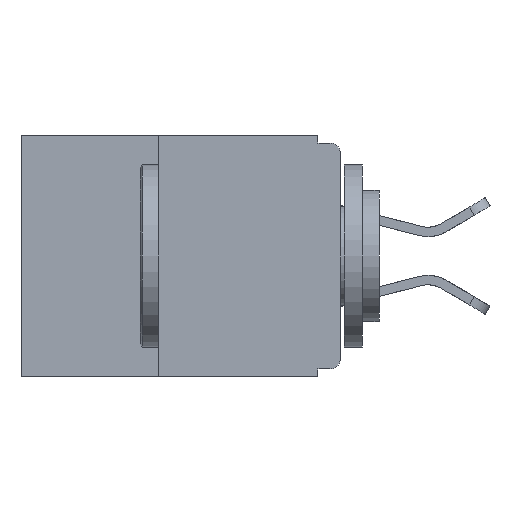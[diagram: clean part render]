
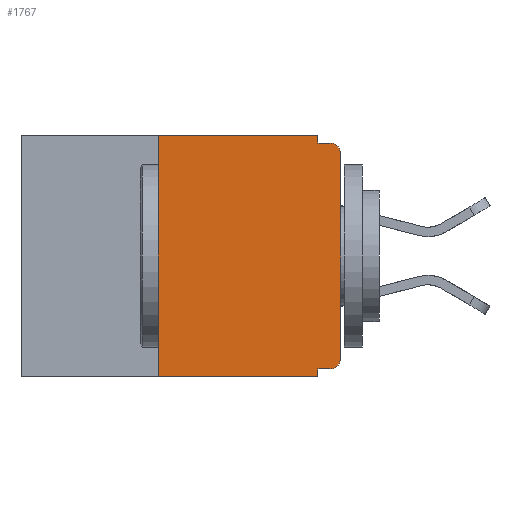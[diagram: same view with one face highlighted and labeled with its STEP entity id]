
A CAD part, left-side view. The second image highlights one B-rep face of the part: STEP entity #1767.
In plain terms, the highlighted planar face has unit normal (-1, 0, 0).
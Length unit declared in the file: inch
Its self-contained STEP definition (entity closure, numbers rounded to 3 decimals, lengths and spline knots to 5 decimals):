
#388 = ORIENTED_EDGE ( 'NONE', *, *, #21669, .T. ) ;
#803 = AXIS2_PLACEMENT_3D ( 'NONE', #18726, #20432, #6730 ) ;
#1104 = EDGE_CURVE ( 'NONE', #9653, #21299, #22819, .T. ) ;
#1432 = CARTESIAN_POINT ( 'NONE',  ( 0., 0.031, -0.32 ) ) ;
#1767 = ADVANCED_FACE ( 'NONE', ( #17740 ), #26815, .F. ) ;
#2661 = EDGE_CURVE ( 'NONE', #14285, #3404, #26125, .T. ) ;
#3115 = CARTESIAN_POINT ( 'NONE',  ( 0., 0.031, -0.01 ) ) ;
#3314 = ORIENTED_EDGE ( 'NONE', *, *, #5586, .F. ) ;
#3404 = VERTEX_POINT ( 'NONE', #3115 ) ;
#4456 = CARTESIAN_POINT ( 'NONE',  ( 0., 0.015, -0.025 ) ) ;
#4927 = VECTOR ( 'NONE', #9873, 39.37008 ) ;
#5070 = ORIENTED_EDGE ( 'NONE', *, *, #2661, .F. ) ;
#5586 = EDGE_CURVE ( 'NONE', #3404, #8520, #14780, .T. ) ;
#5898 = ORIENTED_EDGE ( 'NONE', *, *, #29125, .F. ) ;
#5995 = AXIS2_PLACEMENT_3D ( 'NONE', #4456, #20615, #6744 ) ;
#6149 = ORIENTED_EDGE ( 'NONE', *, *, #1104, .F. ) ;
#6300 = DIRECTION ( 'NONE',  ( 0., 0., 1. ) ) ;
#6730 = DIRECTION ( 'NONE',  ( 0., 0., -1. ) ) ;
#6744 = DIRECTION ( 'NONE',  ( 0., 0., -1. ) ) ;
#6872 = CARTESIAN_POINT ( 'NONE',  ( 0., 0.25, 0. ) ) ;
#6942 = ORIENTED_EDGE ( 'NONE', *, *, #29379, .T. ) ;
#7044 = ORIENTED_EDGE ( 'NONE', *, *, #27943, .F. ) ;
#7077 = VERTEX_POINT ( 'NONE', #13948 ) ;
#7423 = ORIENTED_EDGE ( 'NONE', *, *, #26264, .F. ) ;
#7682 = VECTOR ( 'NONE', #28494, 39.37008 ) ;
#7855 = VECTOR ( 'NONE', #14059, 39.37008 ) ;
#7862 = ORIENTED_EDGE ( 'NONE', *, *, #18554, .T. ) ;
#7995 = VERTEX_POINT ( 'NONE', #1432 ) ;
#8294 = CARTESIAN_POINT ( 'NONE',  ( 0., 0.015, -0.305 ) ) ;
#8520 = VERTEX_POINT ( 'NONE', #12567 ) ;
#9653 = VERTEX_POINT ( 'NONE', #16827 ) ;
#9873 = DIRECTION ( 'NONE',  ( 0., -1., 0. ) ) ;
#9968 = VERTEX_POINT ( 'NONE', #22779 ) ;
#10197 = LINE ( 'NONE', #22814, #27810 ) ;
#10354 = LINE ( 'NONE', #21405, #4927 ) ;
#10688 = DIRECTION ( 'NONE',  ( 0., 0., -1. ) ) ;
#11153 = CARTESIAN_POINT ( 'NONE',  ( 0., 0.25, -0.33 ) ) ;
#11545 = VECTOR ( 'NONE', #18148, 39.37008 ) ;
#11812 = EDGE_CURVE ( 'NONE', #14711, #9968, #18597, .T. ) ;
#12180 = LINE ( 'NONE', #25023, #25155 ) ;
#12276 = LINE ( 'NONE', #27364, #11545 ) ;
#12567 = CARTESIAN_POINT ( 'NONE',  ( 0., 0.015, -0.01 ) ) ;
#13948 = CARTESIAN_POINT ( 'NONE',  ( 0., 0.015, -0.32 ) ) ;
#14059 = DIRECTION ( 'NONE',  ( 0., -1., 0. ) ) ;
#14088 = VERTEX_POINT ( 'NONE', #23861 ) ;
#14214 = CARTESIAN_POINT ( 'NONE',  ( 0., 0., -0.01 ) ) ;
#14285 = VERTEX_POINT ( 'NONE', #24553 ) ;
#14584 = EDGE_LOOP ( 'NONE', ( #14592, #388, #3314, #5070, #5898, #6149, #6942, #7044, #7423, #7862 ) ) ;
#14592 = ORIENTED_EDGE ( 'NONE', *, *, #11812, .T. ) ;
#14711 = VERTEX_POINT ( 'NONE', #26333 ) ;
#14780 = LINE ( 'NONE', #14214, #7855 ) ;
#16688 = VECTOR ( 'NONE', #25220, 39.37008 ) ;
#16827 = CARTESIAN_POINT ( 'NONE',  ( 0., 0.25, -0.33 ) ) ;
#17740 = FACE_OUTER_BOUND ( 'NONE', #14584, .T. ) ;
#18148 = DIRECTION ( 'NONE',  ( 0., 0., -1. ) ) ;
#18554 = EDGE_CURVE ( 'NONE', #7077, #14711, #22226, .T. ) ;
#18597 = LINE ( 'NONE', #22475, #24023 ) ;
#18726 = CARTESIAN_POINT ( 'NONE',  ( 0., 0.437, 0. ) ) ;
#20432 = DIRECTION ( 'NONE',  ( 1., 0., 0. ) ) ;
#20615 = DIRECTION ( 'NONE',  ( -1., 0., 0. ) ) ;
#21299 = VERTEX_POINT ( 'NONE', #6872 ) ;
#21405 = CARTESIAN_POINT ( 'NONE',  ( 0., 0.437, -0.33 ) ) ;
#21669 = EDGE_CURVE ( 'NONE', #9968, #8520, #23126, .T. ) ;
#22226 = CIRCLE ( 'NONE', #24722, 0.015 ) ;
#22475 = CARTESIAN_POINT ( 'NONE',  ( 0., 0., 0. ) ) ;
#22779 = CARTESIAN_POINT ( 'NONE',  ( 0., 0., -0.025 ) ) ;
#22814 = CARTESIAN_POINT ( 'NONE',  ( 0., 0., -0.32 ) ) ;
#22819 = LINE ( 'NONE', #11153, #16688 ) ;
#23126 = CIRCLE ( 'NONE', #5995, 0.015 ) ;
#23861 = CARTESIAN_POINT ( 'NONE',  ( 0., 0.031, -0.33 ) ) ;
#24023 = VECTOR ( 'NONE', #6300, 39.37008 ) ;
#24503 = DIRECTION ( 'NONE',  ( -1., 0., 0. ) ) ;
#24553 = CARTESIAN_POINT ( 'NONE',  ( 0., 0.031, 0. ) ) ;
#24722 = AXIS2_PLACEMENT_3D ( 'NONE', #8294, #24503, #10688 ) ;
#25023 = CARTESIAN_POINT ( 'NONE',  ( 0., 0.437, 0. ) ) ;
#25136 = DIRECTION ( 'NONE',  ( 0., 1., 0. ) ) ;
#25155 = VECTOR ( 'NONE', #27297, 39.37008 ) ;
#25220 = DIRECTION ( 'NONE',  ( 0., 0., 1. ) ) ;
#26125 = LINE ( 'NONE', #28653, #7682 ) ;
#26264 = EDGE_CURVE ( 'NONE', #7077, #7995, #10197, .T. ) ;
#26333 = CARTESIAN_POINT ( 'NONE',  ( 0., 0., -0.305 ) ) ;
#26815 = PLANE ( 'NONE',  #803 ) ;
#27297 = DIRECTION ( 'NONE',  ( 0., -1., 0. ) ) ;
#27364 = CARTESIAN_POINT ( 'NONE',  ( 0., 0.031, -0.33 ) ) ;
#27810 = VECTOR ( 'NONE', #25136, 39.37008 ) ;
#27943 = EDGE_CURVE ( 'NONE', #7995, #14088, #12276, .T. ) ;
#28494 = DIRECTION ( 'NONE',  ( 0., 0., -1. ) ) ;
#28653 = CARTESIAN_POINT ( 'NONE',  ( 0., 0.031, 0. ) ) ;
#29125 = EDGE_CURVE ( 'NONE', #21299, #14285, #12180, .T. ) ;
#29379 = EDGE_CURVE ( 'NONE', #9653, #14088, #10354, .T. ) ;
